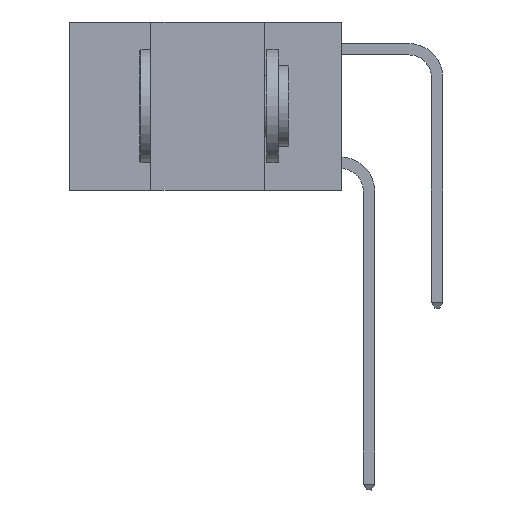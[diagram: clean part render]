
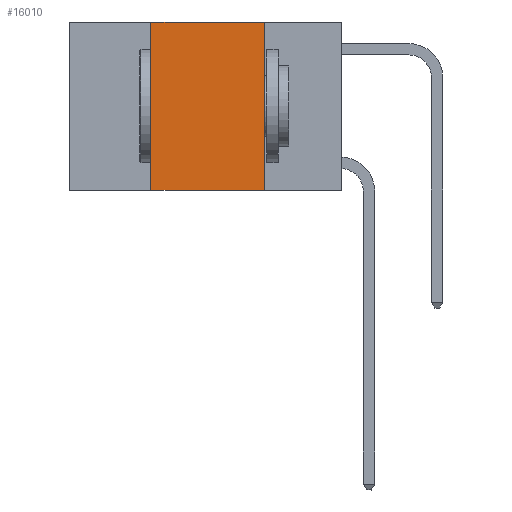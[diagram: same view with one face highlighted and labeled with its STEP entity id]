
A CAD part, left-side view. The second image highlights one B-rep face of the part: STEP entity #16010.
In plain terms, the highlighted planar face has unit normal (-1, 0, 0).
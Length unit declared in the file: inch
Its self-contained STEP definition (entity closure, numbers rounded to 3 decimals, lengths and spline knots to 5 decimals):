
#103 = LINE ( 'NONE', #8255, #8498 ) ;
#275 = LINE ( 'NONE', #2422, #13091 ) ;
#1609 = VERTEX_POINT ( 'NONE', #12593 ) ;
#1893 = ORIENTED_EDGE ( 'NONE', *, *, #9536, .F. ) ;
#2422 = CARTESIAN_POINT ( 'NONE',  ( 0., 0.17, 0. ) ) ;
#3574 = LINE ( 'NONE', #11989, #8846 ) ;
#3891 = EDGE_CURVE ( 'NONE', #15934, #26582, #3574, .T. ) ;
#4768 = CARTESIAN_POINT ( 'NONE',  ( 0., 0.42, -0.37 ) ) ;
#5176 = FACE_OUTER_BOUND ( 'NONE', #21301, .T. ) ;
#7985 = DIRECTION ( 'NONE',  ( 0., -1., 0. ) ) ;
#8255 = CARTESIAN_POINT ( 'NONE',  ( 0., 0.6, -0.37 ) ) ;
#8498 = VECTOR ( 'NONE', #7985, 39.37008 ) ;
#8846 = VECTOR ( 'NONE', #20282, 39.37008 ) ;
#9382 = PLANE ( 'NONE',  #24007 ) ;
#9516 = CARTESIAN_POINT ( 'NONE',  ( 0., 0.6, 0. ) ) ;
#9536 = EDGE_CURVE ( 'NONE', #26582, #10231, #14741, .T. ) ;
#10024 = CARTESIAN_POINT ( 'NONE',  ( 0., 0.42, 0. ) ) ;
#10231 = VERTEX_POINT ( 'NONE', #21928 ) ;
#11989 = CARTESIAN_POINT ( 'NONE',  ( 0., 0.42, 0. ) ) ;
#12593 = CARTESIAN_POINT ( 'NONE',  ( 0., 0.17, -0.37 ) ) ;
#12656 = EDGE_CURVE ( 'NONE', #10231, #1609, #275, .T. ) ;
#13091 = VECTOR ( 'NONE', #19009, 39.37008 ) ;
#14741 = LINE ( 'NONE', #19367, #15582 ) ;
#15582 = VECTOR ( 'NONE', #23424, 39.37008 ) ;
#15647 = DIRECTION ( 'NONE',  ( 1., 0., 0. ) ) ;
#15934 = VERTEX_POINT ( 'NONE', #4768 ) ;
#15940 = ORIENTED_EDGE ( 'NONE', *, *, #17909, .T. ) ;
#16010 = ADVANCED_FACE ( 'NONE', ( #5176 ), #9382, .F. ) ;
#17909 = EDGE_CURVE ( 'NONE', #15934, #1609, #103, .T. ) ;
#19009 = DIRECTION ( 'NONE',  ( 0., 0., -1. ) ) ;
#19367 = CARTESIAN_POINT ( 'NONE',  ( 0., 0.6, 0. ) ) ;
#20282 = DIRECTION ( 'NONE',  ( 0., 0., 1. ) ) ;
#20402 = ORIENTED_EDGE ( 'NONE', *, *, #12656, .F. ) ;
#21301 = EDGE_LOOP ( 'NONE', ( #20402, #1893, #22585, #15940 ) ) ;
#21928 = CARTESIAN_POINT ( 'NONE',  ( 0., 0.17, 0. ) ) ;
#22585 = ORIENTED_EDGE ( 'NONE', *, *, #3891, .F. ) ;
#23424 = DIRECTION ( 'NONE',  ( 0., -1., 0. ) ) ;
#24007 = AXIS2_PLACEMENT_3D ( 'NONE', #9516, #15647, #25827 ) ;
#25827 = DIRECTION ( 'NONE',  ( 0., 0., -1. ) ) ;
#26582 = VERTEX_POINT ( 'NONE', #10024 ) ;
